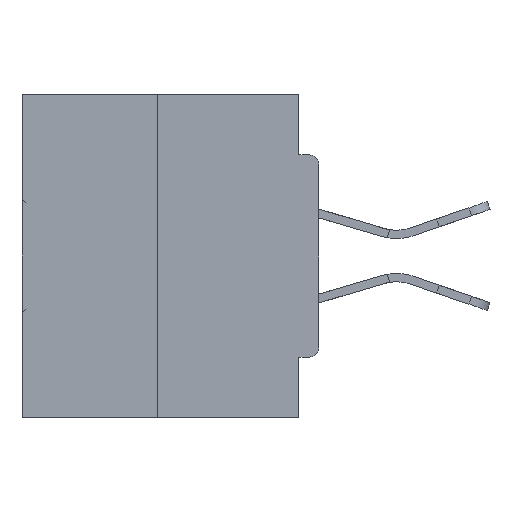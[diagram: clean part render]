
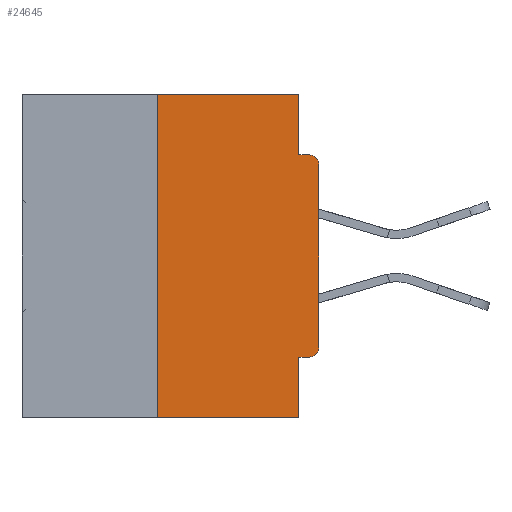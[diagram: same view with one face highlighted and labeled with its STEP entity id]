
A CAD part, left-side view. The second image highlights one B-rep face of the part: STEP entity #24645.
In plain terms, the highlighted planar face has unit normal (-1, 0, 0).
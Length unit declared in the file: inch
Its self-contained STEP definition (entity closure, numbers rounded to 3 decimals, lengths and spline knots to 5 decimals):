
#1341 = DIRECTION ( 'NONE',  ( 0., 0., -1. ) ) ;
#1342 = CARTESIAN_POINT ( 'NONE',  ( 0., 0., -0.4065 ) ) ;
#2296 = EDGE_CURVE ( 'NONE', #20175, #25931, #40774, .T. ) ;
#2351 = CARTESIAN_POINT ( 'NONE',  ( 0., 0.015, -0.4065 ) ) ;
#2451 = VERTEX_POINT ( 'NONE', #20541 ) ;
#2802 = DIRECTION ( 'NONE',  ( 0., -1., 0. ) ) ;
#3165 = DIRECTION ( 'NONE',  ( 0., -1., 0. ) ) ;
#3249 = AXIS2_PLACEMENT_3D ( 'NONE', #6974, #3288, #1341 ) ;
#3288 = DIRECTION ( 'NONE',  ( -1., 0., 0. ) ) ;
#3774 = CIRCLE ( 'NONE', #31896, 0.015 ) ;
#3942 = VECTOR ( 'NONE', #7130, 39.37008 ) ;
#3951 = CARTESIAN_POINT ( 'NONE',  ( 0., 0.015, -0.0935 ) ) ;
#4025 = DIRECTION ( 'NONE',  ( -1., 0., 0. ) ) ;
#5707 = EDGE_CURVE ( 'NONE', #7622, #14930, #17319, .T. ) ;
#6439 = CARTESIAN_POINT ( 'NONE',  ( 0., 0.25, 0. ) ) ;
#6474 = ORIENTED_EDGE ( 'NONE', *, *, #5707, .F. ) ;
#6974 = CARTESIAN_POINT ( 'NONE',  ( 0., 0.015, -0.3915 ) ) ;
#7130 = DIRECTION ( 'NONE',  ( 0., 0., 1. ) ) ;
#7406 = VECTOR ( 'NONE', #2802, 39.37008 ) ;
#7496 = VECTOR ( 'NONE', #42730, 39.37008 ) ;
#7622 = VERTEX_POINT ( 'NONE', #26835 ) ;
#9384 = LINE ( 'NONE', #1342, #38885 ) ;
#10654 = EDGE_CURVE ( 'NONE', #14227, #22653, #25215, .T. ) ;
#11227 = LINE ( 'NONE', #16251, #33852 ) ;
#11295 = ORIENTED_EDGE ( 'NONE', *, *, #16440, .F. ) ;
#12627 = VECTOR ( 'NONE', #15572, 39.37008 ) ;
#13616 = DIRECTION ( 'NONE',  ( 0., 0., 1. ) ) ;
#14077 = CARTESIAN_POINT ( 'NONE',  ( 0., 0.46, 0. ) ) ;
#14227 = VERTEX_POINT ( 'NONE', #2351 ) ;
#14547 = AXIS2_PLACEMENT_3D ( 'NONE', #14077, #38237, #18035 ) ;
#14930 = VERTEX_POINT ( 'NONE', #3951 ) ;
#14939 = VERTEX_POINT ( 'NONE', #36793 ) ;
#15255 = ORIENTED_EDGE ( 'NONE', *, *, #29967, .T. ) ;
#15572 = DIRECTION ( 'NONE',  ( 0., -1., 0. ) ) ;
#15765 = CARTESIAN_POINT ( 'NONE',  ( 0., 0.031, -0.5 ) ) ;
#16251 = CARTESIAN_POINT ( 'NONE',  ( 0., 0.031, 0. ) ) ;
#16419 = LINE ( 'NONE', #15765, #7496 ) ;
#16440 = EDGE_CURVE ( 'NONE', #14227, #2451, #9384, .T. ) ;
#17319 = LINE ( 'NONE', #28948, #12627 ) ;
#18035 = DIRECTION ( 'NONE',  ( 0., 0., -1. ) ) ;
#18268 = EDGE_CURVE ( 'NONE', #22653, #14939, #25032, .T. ) ;
#19247 = EDGE_CURVE ( 'NONE', #22293, #7622, #11227, .T. ) ;
#19547 = EDGE_CURVE ( 'NONE', #2451, #29121, #16419, .T. ) ;
#19696 = VECTOR ( 'NONE', #13616, 39.37008 ) ;
#20175 = VERTEX_POINT ( 'NONE', #28896 ) ;
#20541 = CARTESIAN_POINT ( 'NONE',  ( 0., 0.031, -0.4065 ) ) ;
#20952 = DIRECTION ( 'NONE',  ( 0., 0., -1. ) ) ;
#21960 = ORIENTED_EDGE ( 'NONE', *, *, #19547, .F. ) ;
#22293 = VERTEX_POINT ( 'NONE', #29938 ) ;
#22653 = VERTEX_POINT ( 'NONE', #30181 ) ;
#22947 = CARTESIAN_POINT ( 'NONE',  ( 0., 0.46, -0.5 ) ) ;
#23321 = CARTESIAN_POINT ( 'NONE',  ( 0., 0.46, 0. ) ) ;
#24484 = CARTESIAN_POINT ( 'NONE',  ( 0., 0.015, -0.1085 ) ) ;
#24645 = ADVANCED_FACE ( 'NONE', ( #39765 ), #38081, .F. ) ;
#25032 = LINE ( 'NONE', #33910, #3942 ) ;
#25215 = CIRCLE ( 'NONE', #3249, 0.015 ) ;
#25931 = VERTEX_POINT ( 'NONE', #42475 ) ;
#26835 = CARTESIAN_POINT ( 'NONE',  ( 0., 0.031, -0.0935 ) ) ;
#27085 = LINE ( 'NONE', #23321, #35035 ) ;
#28896 = CARTESIAN_POINT ( 'NONE',  ( 0., 0.25, -0.5 ) ) ;
#28948 = CARTESIAN_POINT ( 'NONE',  ( 0., 0., -0.0935 ) ) ;
#29121 = VERTEX_POINT ( 'NONE', #32110 ) ;
#29938 = CARTESIAN_POINT ( 'NONE',  ( 0., 0.031, 0. ) ) ;
#29967 = EDGE_CURVE ( 'NONE', #14939, #14930, #3774, .T. ) ;
#30181 = CARTESIAN_POINT ( 'NONE',  ( 0., 0., -0.3915 ) ) ;
#31286 = ORIENTED_EDGE ( 'NONE', *, *, #10654, .T. ) ;
#31896 = AXIS2_PLACEMENT_3D ( 'NONE', #24484, #4025, #20952 ) ;
#32110 = CARTESIAN_POINT ( 'NONE',  ( 0., 0.031, -0.5 ) ) ;
#33719 = LINE ( 'NONE', #22947, #7406 ) ;
#33852 = VECTOR ( 'NONE', #36388, 39.37008 ) ;
#33910 = CARTESIAN_POINT ( 'NONE',  ( 0., 0., 0. ) ) ;
#35035 = VECTOR ( 'NONE', #3165, 39.37008 ) ;
#36388 = DIRECTION ( 'NONE',  ( 0., 0., -1. ) ) ;
#36793 = CARTESIAN_POINT ( 'NONE',  ( 0., 0., -0.1085 ) ) ;
#37990 = DIRECTION ( 'NONE',  ( 0., 1., 0. ) ) ;
#38013 = EDGE_CURVE ( 'NONE', #25931, #22293, #27085, .T. ) ;
#38081 = PLANE ( 'NONE',  #14547 ) ;
#38237 = DIRECTION ( 'NONE',  ( 1., 0., 0. ) ) ;
#38766 = ORIENTED_EDGE ( 'NONE', *, *, #41043, .T. ) ;
#38885 = VECTOR ( 'NONE', #37990, 39.37008 ) ;
#39276 = ORIENTED_EDGE ( 'NONE', *, *, #2296, .F. ) ;
#39765 = FACE_OUTER_BOUND ( 'NONE', #41431, .T. ) ;
#40350 = ORIENTED_EDGE ( 'NONE', *, *, #18268, .T. ) ;
#40534 = ORIENTED_EDGE ( 'NONE', *, *, #19247, .F. ) ;
#40774 = LINE ( 'NONE', #6439, #19696 ) ;
#41043 = EDGE_CURVE ( 'NONE', #20175, #29121, #33719, .T. ) ;
#41431 = EDGE_LOOP ( 'NONE', ( #43506, #39276, #38766, #21960, #11295, #31286, #40350, #15255, #6474, #40534 ) ) ;
#42475 = CARTESIAN_POINT ( 'NONE',  ( 0., 0.25, 0. ) ) ;
#42730 = DIRECTION ( 'NONE',  ( 0., 0., -1. ) ) ;
#43506 = ORIENTED_EDGE ( 'NONE', *, *, #38013, .F. ) ;
